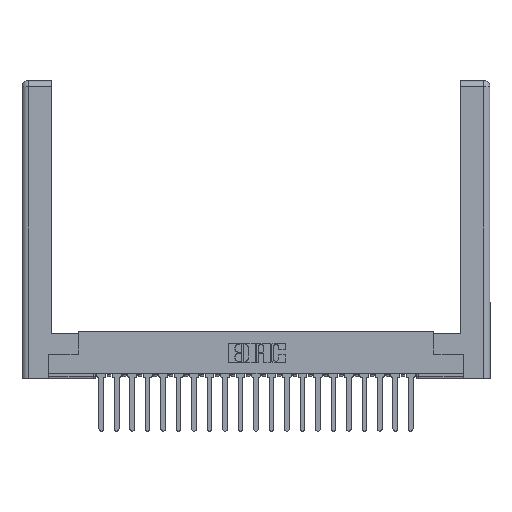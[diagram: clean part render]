
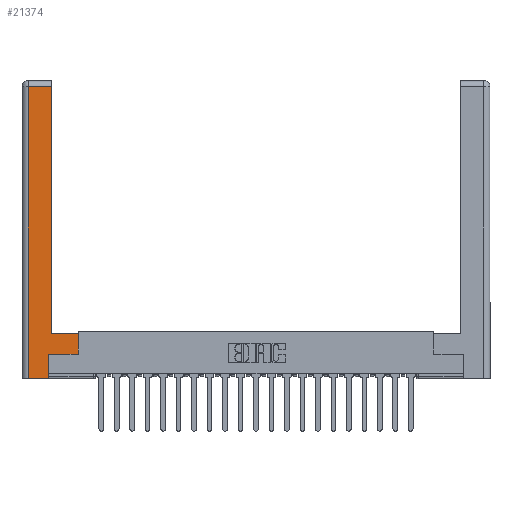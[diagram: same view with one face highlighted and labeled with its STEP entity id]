
A CAD part, top view. The second image highlights one B-rep face of the part: STEP entity #21374.
In plain terms, the highlighted planar face has unit normal (0, 0, 1).
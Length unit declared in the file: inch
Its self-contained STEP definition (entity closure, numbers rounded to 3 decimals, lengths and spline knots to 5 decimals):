
#278 = FACE_OUTER_BOUND ( 'NONE', #14576, .T. ) ;
#383 = VERTEX_POINT ( 'NONE', #14526 ) ;
#873 = VECTOR ( 'NONE', #3366, 39.37008 ) ;
#2352 = DIRECTION ( 'NONE',  ( -1., 0., 0. ) ) ;
#3104 = EDGE_CURVE ( 'NONE', #22567, #15354, #13665, .T. ) ;
#3215 = CARTESIAN_POINT ( 'NONE',  ( 0.295, 3., 0. ) ) ;
#3366 = DIRECTION ( 'NONE',  ( 0., 1., 0. ) ) ;
#3421 = VERTEX_POINT ( 'NONE', #3637 ) ;
#3425 = CARTESIAN_POINT ( 'NONE',  ( 0.265, 0.245, 0. ) ) ;
#3565 = LINE ( 'NONE', #3215, #22054 ) ;
#3637 = CARTESIAN_POINT ( 'NONE',  ( 0.0615, 2.94, 0. ) ) ;
#4122 = CARTESIAN_POINT ( 'NONE',  ( 0.0615, 0., 0. ) ) ;
#4188 = VECTOR ( 'NONE', #17419, 39.37008 ) ;
#4236 = CARTESIAN_POINT ( 'NONE',  ( 0.0615, 0., 0. ) ) ;
#4850 = DIRECTION ( 'NONE',  ( 1., 0., 0. ) ) ;
#4955 = VECTOR ( 'NONE', #20671, 39.37008 ) ;
#4975 = LINE ( 'NONE', #14489, #5507 ) ;
#5184 = CARTESIAN_POINT ( 'NONE',  ( 0.265, 0.245, 0. ) ) ;
#5278 = EDGE_CURVE ( 'NONE', #6374, #22567, #23122, .T. ) ;
#5336 = ORIENTED_EDGE ( 'NONE', *, *, #20043, .T. ) ;
#5500 = DIRECTION ( 'NONE',  ( 0., 1., 0. ) ) ;
#5507 = VECTOR ( 'NONE', #4850, 39.37008 ) ;
#5700 = VERTEX_POINT ( 'NONE', #4122 ) ;
#6311 = EDGE_CURVE ( 'NONE', #15354, #18139, #3565, .T. ) ;
#6374 = VERTEX_POINT ( 'NONE', #19773 ) ;
#6558 = DIRECTION ( 'NONE',  ( 0., 1., 0. ) ) ;
#6619 = VERTEX_POINT ( 'NONE', #3425 ) ;
#7051 = CARTESIAN_POINT ( 'NONE',  ( 0.295, 2.94, 0. ) ) ;
#7163 = EDGE_CURVE ( 'NONE', #6619, #6374, #4975, .T. ) ;
#7401 = ORIENTED_EDGE ( 'NONE', *, *, #13211, .T. ) ;
#7612 = EDGE_CURVE ( 'NONE', #383, #6619, #21742, .T. ) ;
#7651 = PLANE ( 'NONE',  #10366 ) ;
#8242 = CARTESIAN_POINT ( 'NONE',  ( 0.565, 0.45, 0. ) ) ;
#8514 = CARTESIAN_POINT ( 'NONE',  ( 0.265, 0., 0. ) ) ;
#9048 = EDGE_CURVE ( 'NONE', #5700, #383, #19513, .T. ) ;
#9467 = VECTOR ( 'NONE', #11756, 39.37008 ) ;
#10366 = AXIS2_PLACEMENT_3D ( 'NONE', #15017, #22399, #13192 ) ;
#11089 = ORIENTED_EDGE ( 'NONE', *, *, #9048, .T. ) ;
#11756 = DIRECTION ( 'NONE',  ( 1., 0., 0. ) ) ;
#13192 = DIRECTION ( 'NONE',  ( -1., 0., 0. ) ) ;
#13211 = EDGE_CURVE ( 'NONE', #18139, #3421, #18902, .T. ) ;
#13336 = ORIENTED_EDGE ( 'NONE', *, *, #7163, .T. ) ;
#13665 = LINE ( 'NONE', #18887, #4188 ) ;
#13894 = ORIENTED_EDGE ( 'NONE', *, *, #6311, .T. ) ;
#14261 = ORIENTED_EDGE ( 'NONE', *, *, #5278, .T. ) ;
#14489 = CARTESIAN_POINT ( 'NONE',  ( 0.565, 0.245, 0. ) ) ;
#14526 = CARTESIAN_POINT ( 'NONE',  ( 0.265, 0., 0. ) ) ;
#14576 = EDGE_LOOP ( 'NONE', ( #13894, #7401, #5336, #11089, #19919, #13336, #14261, #14595 ) ) ;
#14595 = ORIENTED_EDGE ( 'NONE', *, *, #3104, .T. ) ;
#15017 = CARTESIAN_POINT ( 'NONE',  ( 0., 0., 0. ) ) ;
#15354 = VERTEX_POINT ( 'NONE', #20543 ) ;
#16727 = CARTESIAN_POINT ( 'NONE',  ( 0.0615, 2.94, 0. ) ) ;
#17419 = DIRECTION ( 'NONE',  ( -1., 0., 0. ) ) ;
#18139 = VERTEX_POINT ( 'NONE', #7051 ) ;
#18887 = CARTESIAN_POINT ( 'NONE',  ( 0.295, 0.45, 0. ) ) ;
#18902 = LINE ( 'NONE', #16727, #18949 ) ;
#18949 = VECTOR ( 'NONE', #2352, 39.37008 ) ;
#19513 = LINE ( 'NONE', #8514, #9467 ) ;
#19773 = CARTESIAN_POINT ( 'NONE',  ( 0.565, 0.245, 0. ) ) ;
#19919 = ORIENTED_EDGE ( 'NONE', *, *, #7612, .T. ) ;
#20043 = EDGE_CURVE ( 'NONE', #3421, #5700, #22596, .T. ) ;
#20543 = CARTESIAN_POINT ( 'NONE',  ( 0.295, 0.45, 0. ) ) ;
#20671 = DIRECTION ( 'NONE',  ( 0., -1., 0. ) ) ;
#21374 = ADVANCED_FACE ( 'NONE', ( #278 ), #7651, .F. ) ;
#21742 = LINE ( 'NONE', #5184, #873 ) ;
#22054 = VECTOR ( 'NONE', #5500, 39.37008 ) ;
#22399 = DIRECTION ( 'NONE',  ( 0., 0., -1. ) ) ;
#22567 = VERTEX_POINT ( 'NONE', #22929 ) ;
#22596 = LINE ( 'NONE', #4236, #4955 ) ;
#22929 = CARTESIAN_POINT ( 'NONE',  ( 0.565, 0.45, 0. ) ) ;
#23122 = LINE ( 'NONE', #8242, #23572 ) ;
#23572 = VECTOR ( 'NONE', #6558, 39.37008 ) ;
